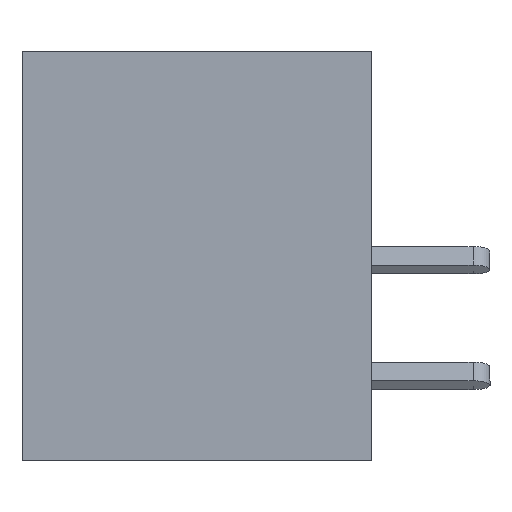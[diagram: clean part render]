
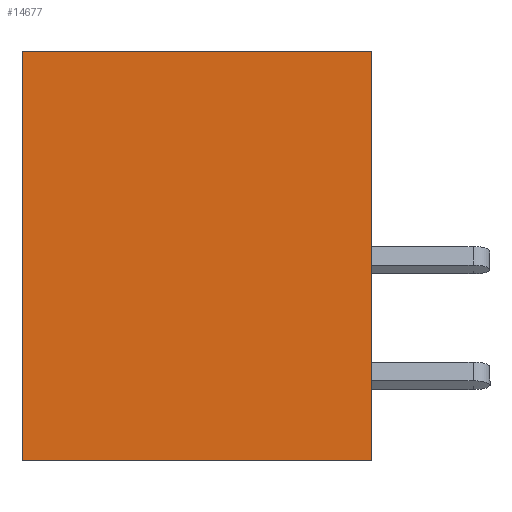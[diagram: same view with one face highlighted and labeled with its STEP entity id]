
A CAD part, left-side view. The second image highlights one B-rep face of the part: STEP entity #14677.
In plain terms, the highlighted planar face has unit normal (-1, 0, 0).
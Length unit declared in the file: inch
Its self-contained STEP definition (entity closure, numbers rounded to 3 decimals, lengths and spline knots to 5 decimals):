
#110 = AXIS2_PLACEMENT_3D ( 'NONE', #13541, #24373, #5167 ) ;
#1517 = VERTEX_POINT ( 'NONE', #10053 ) ;
#1599 = CARTESIAN_POINT ( 'NONE',  ( 0., 0.453, 0. ) ) ;
#1793 = DIRECTION ( 'NONE',  ( 0., -1., 0. ) ) ;
#2789 = DIRECTION ( 'NONE',  ( 0., 0., 1. ) ) ;
#5167 = DIRECTION ( 'NONE',  ( 0., 0., -1. ) ) ;
#5763 = ORIENTED_EDGE ( 'NONE', *, *, #16272, .F. ) ;
#7217 = LINE ( 'NONE', #1599, #9524 ) ;
#7974 = CARTESIAN_POINT ( 'NONE',  ( 0., 0.453, 0. ) ) ;
#8517 = CARTESIAN_POINT ( 'NONE',  ( 0., 0.453, -0.531 ) ) ;
#8880 = EDGE_CURVE ( 'NONE', #1517, #9639, #23532, .T. ) ;
#9343 = PLANE ( 'NONE',  #110 ) ;
#9524 = VECTOR ( 'NONE', #1793, 39.37008 ) ;
#9639 = VERTEX_POINT ( 'NONE', #19997 ) ;
#10053 = CARTESIAN_POINT ( 'NONE',  ( 0., 0., -0.531 ) ) ;
#10549 = VERTEX_POINT ( 'NONE', #25473 ) ;
#10597 = EDGE_LOOP ( 'NONE', ( #26966, #5763, #11528, #25459 ) ) ;
#11169 = LINE ( 'NONE', #7974, #20603 ) ;
#11271 = FACE_OUTER_BOUND ( 'NONE', #10597, .T. ) ;
#11528 = ORIENTED_EDGE ( 'NONE', *, *, #16664, .F. ) ;
#13541 = CARTESIAN_POINT ( 'NONE',  ( 0., 0.453, 0. ) ) ;
#14125 = DIRECTION ( 'NONE',  ( 0., 0., 1. ) ) ;
#14221 = LINE ( 'NONE', #8517, #27351 ) ;
#14677 = ADVANCED_FACE ( 'NONE', ( #11271 ), #9343, .F. ) ;
#16272 = EDGE_CURVE ( 'NONE', #26913, #9639, #7217, .T. ) ;
#16664 = EDGE_CURVE ( 'NONE', #10549, #26913, #11169, .T. ) ;
#19997 = CARTESIAN_POINT ( 'NONE',  ( 0., 0., 0. ) ) ;
#20277 = EDGE_CURVE ( 'NONE', #10549, #1517, #14221, .T. ) ;
#20603 = VECTOR ( 'NONE', #14125, 39.37008 ) ;
#23532 = LINE ( 'NONE', #23982, #24190 ) ;
#23982 = CARTESIAN_POINT ( 'NONE',  ( 0., 0., 0. ) ) ;
#24190 = VECTOR ( 'NONE', #2789, 39.37008 ) ;
#24373 = DIRECTION ( 'NONE',  ( 1., 0., 0. ) ) ;
#25459 = ORIENTED_EDGE ( 'NONE', *, *, #20277, .T. ) ;
#25473 = CARTESIAN_POINT ( 'NONE',  ( 0., 0.453, -0.531 ) ) ;
#25698 = DIRECTION ( 'NONE',  ( 0., -1., 0. ) ) ;
#26108 = CARTESIAN_POINT ( 'NONE',  ( 0., 0.453, 0. ) ) ;
#26913 = VERTEX_POINT ( 'NONE', #26108 ) ;
#26966 = ORIENTED_EDGE ( 'NONE', *, *, #8880, .T. ) ;
#27351 = VECTOR ( 'NONE', #25698, 39.37008 ) ;
